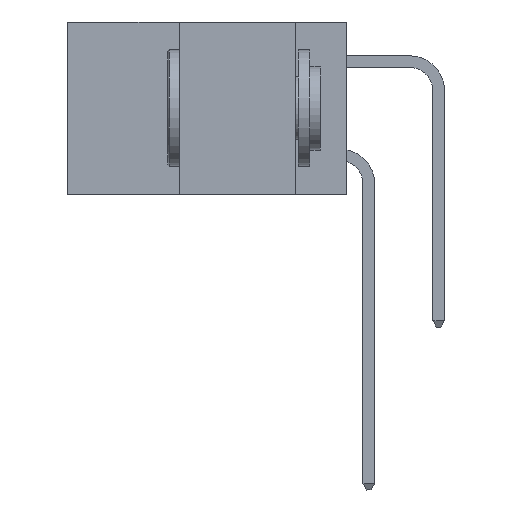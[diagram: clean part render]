
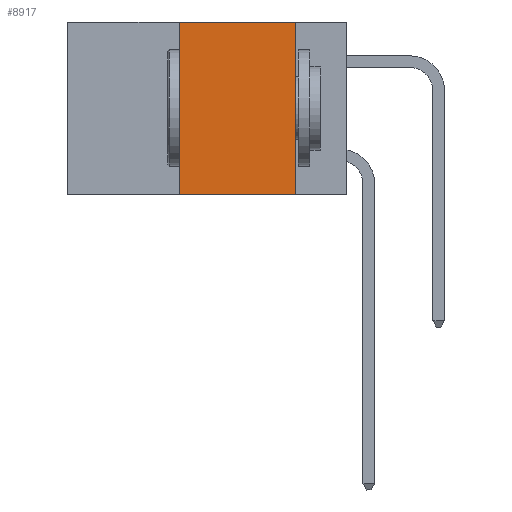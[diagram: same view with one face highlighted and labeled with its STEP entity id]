
A CAD part, left-side view. The second image highlights one B-rep face of the part: STEP entity #8917.
In plain terms, the highlighted planar face has unit normal (-1, 0, 0).
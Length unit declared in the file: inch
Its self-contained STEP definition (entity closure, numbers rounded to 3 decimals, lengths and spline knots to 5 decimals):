
#236 = CARTESIAN_POINT ( 'NONE',  ( 0., 0.11, -0.37 ) ) ;
#1154 = LINE ( 'NONE', #6424, #15269 ) ;
#1424 = DIRECTION ( 'NONE',  ( 0., 0., 1. ) ) ;
#2347 = LINE ( 'NONE', #12480, #2588 ) ;
#2380 = DIRECTION ( 'NONE',  ( 0., 0., -1. ) ) ;
#2588 = VECTOR ( 'NONE', #1424, 39.37008 ) ;
#2769 = ORIENTED_EDGE ( 'NONE', *, *, #11969, .F. ) ;
#3221 = FACE_OUTER_BOUND ( 'NONE', #13888, .T. ) ;
#3726 = CARTESIAN_POINT ( 'NONE',  ( 0., 0.6, 0. ) ) ;
#4167 = AXIS2_PLACEMENT_3D ( 'NONE', #20800, #22660, #11845 ) ;
#4629 = VECTOR ( 'NONE', #2380, 39.37008 ) ;
#6424 = CARTESIAN_POINT ( 'NONE',  ( 0., 0.6, -0.37 ) ) ;
#7032 = VECTOR ( 'NONE', #9563, 39.37008 ) ;
#8246 = DIRECTION ( 'NONE',  ( 0., -1., 0. ) ) ;
#8917 = ADVANCED_FACE ( 'NONE', ( #3221 ), #9969, .F. ) ;
#8919 = CARTESIAN_POINT ( 'NONE',  ( 0., 0.36, 0. ) ) ;
#9507 = LINE ( 'NONE', #22395, #4629 ) ;
#9563 = DIRECTION ( 'NONE',  ( 0., -1., 0. ) ) ;
#9969 = PLANE ( 'NONE',  #4167 ) ;
#11845 = DIRECTION ( 'NONE',  ( 0., 0., -1. ) ) ;
#11969 = EDGE_CURVE ( 'NONE', #19870, #12624, #12526, .T. ) ;
#12480 = CARTESIAN_POINT ( 'NONE',  ( 0., 0.36, 0. ) ) ;
#12526 = LINE ( 'NONE', #3726, #7032 ) ;
#12624 = VERTEX_POINT ( 'NONE', #13442 ) ;
#13442 = CARTESIAN_POINT ( 'NONE',  ( 0., 0.11, 0. ) ) ;
#13888 = EDGE_LOOP ( 'NONE', ( #18699, #2769, #19992, #22701 ) ) ;
#14183 = EDGE_CURVE ( 'NONE', #20492, #19870, #2347, .T. ) ;
#14407 = VERTEX_POINT ( 'NONE', #236 ) ;
#14503 = EDGE_CURVE ( 'NONE', #12624, #14407, #9507, .T. ) ;
#14830 = CARTESIAN_POINT ( 'NONE',  ( 0., 0.36, -0.37 ) ) ;
#15110 = EDGE_CURVE ( 'NONE', #20492, #14407, #1154, .T. ) ;
#15269 = VECTOR ( 'NONE', #8246, 39.37008 ) ;
#18699 = ORIENTED_EDGE ( 'NONE', *, *, #14503, .F. ) ;
#19870 = VERTEX_POINT ( 'NONE', #8919 ) ;
#19992 = ORIENTED_EDGE ( 'NONE', *, *, #14183, .F. ) ;
#20492 = VERTEX_POINT ( 'NONE', #14830 ) ;
#20800 = CARTESIAN_POINT ( 'NONE',  ( 0., 0.6, 0. ) ) ;
#22395 = CARTESIAN_POINT ( 'NONE',  ( 0., 0.11, 0. ) ) ;
#22660 = DIRECTION ( 'NONE',  ( 1., 0., 0. ) ) ;
#22701 = ORIENTED_EDGE ( 'NONE', *, *, #15110, .T. ) ;
